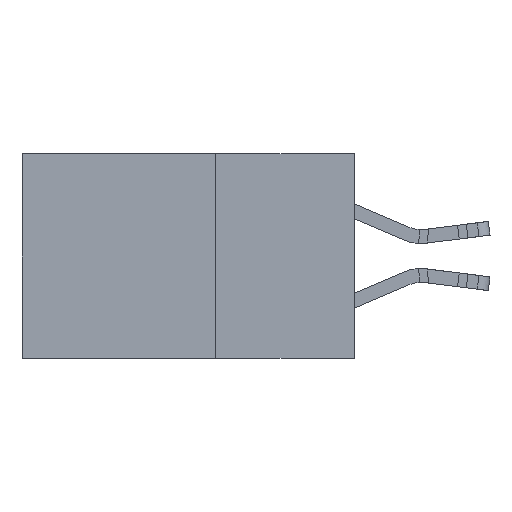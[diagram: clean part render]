
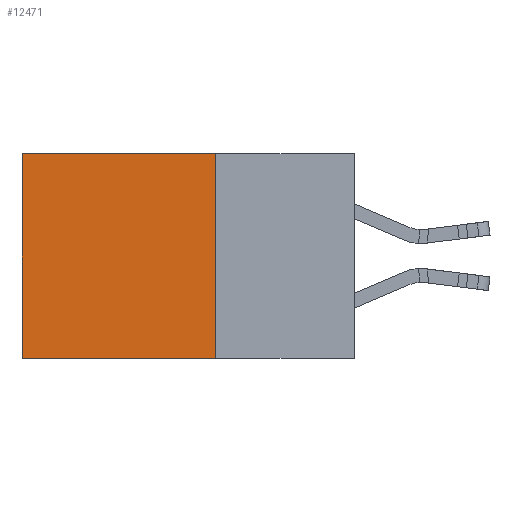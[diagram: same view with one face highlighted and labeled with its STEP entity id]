
A CAD part, left-side view. The second image highlights one B-rep face of the part: STEP entity #12471.
In plain terms, the highlighted planar face has unit normal (-1, 0, 0).
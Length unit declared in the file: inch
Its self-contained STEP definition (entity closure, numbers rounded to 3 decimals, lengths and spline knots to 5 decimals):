
#597 = DIRECTION ( 'NONE',  ( 1., 0., 0. ) ) ;
#1401 = CARTESIAN_POINT ( 'NONE',  ( 0.2615, 0.25, -0.37 ) ) ;
#2182 = VERTEX_POINT ( 'NONE', #1401 ) ;
#2654 = DIRECTION ( 'NONE',  ( 0., 0., -1. ) ) ;
#3127 = CARTESIAN_POINT ( 'NONE',  ( 0.2615, 0.25, -0.37 ) ) ;
#4031 = VERTEX_POINT ( 'NONE', #25246 ) ;
#4212 = LINE ( 'NONE', #12085, #25261 ) ;
#4937 = LINE ( 'NONE', #24306, #15708 ) ;
#4998 = VECTOR ( 'NONE', #10996, 39.37008 ) ;
#5649 = AXIS2_PLACEMENT_3D ( 'NONE', #8072, #597, #2654 ) ;
#7659 = EDGE_CURVE ( 'NONE', #4031, #17395, #4212, .T. ) ;
#7990 = VERTEX_POINT ( 'NONE', #18149 ) ;
#8072 = CARTESIAN_POINT ( 'NONE',  ( 0.2615, 0.25, -0.37 ) ) ;
#9294 = VECTOR ( 'NONE', #19772, 39.37008 ) ;
#9352 = ORIENTED_EDGE ( 'NONE', *, *, #17948, .T. ) ;
#9807 = ORIENTED_EDGE ( 'NONE', *, *, #10218, .F. ) ;
#10218 = EDGE_CURVE ( 'NONE', #7990, #2182, #17457, .T. ) ;
#10996 = DIRECTION ( 'NONE',  ( 0., 1., 0. ) ) ;
#11942 = FACE_OUTER_BOUND ( 'NONE', #22424, .T. ) ;
#12085 = CARTESIAN_POINT ( 'NONE',  ( 0.2615, 0.6, -0.37 ) ) ;
#12202 = PLANE ( 'NONE',  #5649 ) ;
#12471 = ADVANCED_FACE ( 'NONE', ( #11942 ), #12202, .F. ) ;
#13764 = ORIENTED_EDGE ( 'NONE', *, *, #18029, .F. ) ;
#15708 = VECTOR ( 'NONE', #16697, 39.37008 ) ;
#15962 = DIRECTION ( 'NONE',  ( 0., 0., -1. ) ) ;
#16697 = DIRECTION ( 'NONE',  ( 0., 1., 0. ) ) ;
#17395 = VERTEX_POINT ( 'NONE', #20666 ) ;
#17457 = LINE ( 'NONE', #19523, #9294 ) ;
#17948 = EDGE_CURVE ( 'NONE', #7990, #4031, #4937, .T. ) ;
#18029 = EDGE_CURVE ( 'NONE', #2182, #17395, #20688, .T. ) ;
#18149 = CARTESIAN_POINT ( 'NONE',  ( 0.2615, 0.25, 0. ) ) ;
#18568 = ORIENTED_EDGE ( 'NONE', *, *, #7659, .T. ) ;
#19523 = CARTESIAN_POINT ( 'NONE',  ( 0.2615, 0.25, -0.37 ) ) ;
#19772 = DIRECTION ( 'NONE',  ( 0., 0., -1. ) ) ;
#20666 = CARTESIAN_POINT ( 'NONE',  ( 0.2615, 0.6, -0.37 ) ) ;
#20688 = LINE ( 'NONE', #3127, #4998 ) ;
#22424 = EDGE_LOOP ( 'NONE', ( #18568, #13764, #9807, #9352 ) ) ;
#24306 = CARTESIAN_POINT ( 'NONE',  ( 0.2615, 0.25, 0. ) ) ;
#25246 = CARTESIAN_POINT ( 'NONE',  ( 0.2615, 0.6, 0. ) ) ;
#25261 = VECTOR ( 'NONE', #15962, 39.37008 ) ;
